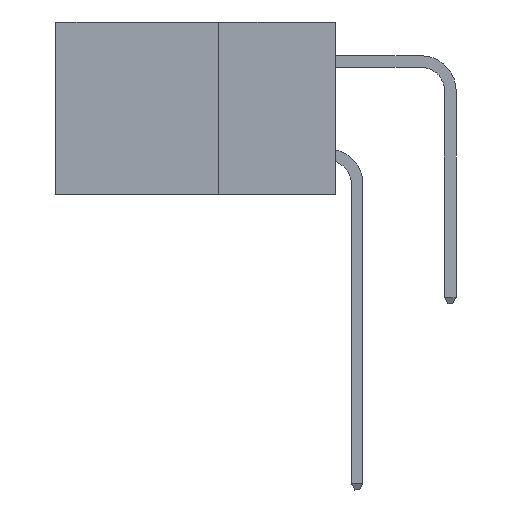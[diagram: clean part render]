
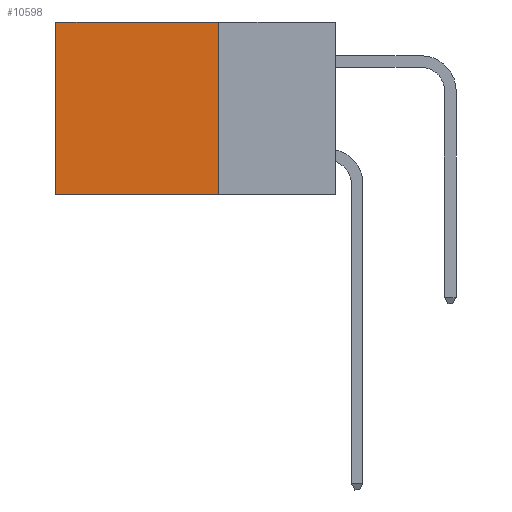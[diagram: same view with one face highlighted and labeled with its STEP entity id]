
A CAD part, left-side view. The second image highlights one B-rep face of the part: STEP entity #10598.
In plain terms, the highlighted planar face has unit normal (-1, 0, 0).
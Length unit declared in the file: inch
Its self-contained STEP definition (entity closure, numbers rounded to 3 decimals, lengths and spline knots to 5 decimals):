
#265 = ORIENTED_EDGE ( 'NONE', *, *, #7087, .T. ) ;
#295 = CARTESIAN_POINT ( 'NONE',  ( 0.2875, 0.6, 0. ) ) ;
#411 = VERTEX_POINT ( 'NONE', #9267 ) ;
#1219 = DIRECTION ( 'NONE',  ( 1., 0., 0. ) ) ;
#1471 = ORIENTED_EDGE ( 'NONE', *, *, #13299, .F. ) ;
#1819 = DIRECTION ( 'NONE',  ( 0., 0., -1. ) ) ;
#2001 = CARTESIAN_POINT ( 'NONE',  ( 0.2875, 0.6, 0. ) ) ;
#3094 = VECTOR ( 'NONE', #5491, 39.37008 ) ;
#3588 = CARTESIAN_POINT ( 'NONE',  ( 0.2875, 0.25, -0.37 ) ) ;
#3976 = CARTESIAN_POINT ( 'NONE',  ( 0.2875, 0.25, -0.37 ) ) ;
#4157 = CARTESIAN_POINT ( 'NONE',  ( 0.2875, 0.25, 0. ) ) ;
#5035 = VERTEX_POINT ( 'NONE', #4157 ) ;
#5067 = LINE ( 'NONE', #17633, #13308 ) ;
#5439 = VERTEX_POINT ( 'NONE', #2001 ) ;
#5491 = DIRECTION ( 'NONE',  ( 0., 1., 0. ) ) ;
#6133 = DIRECTION ( 'NONE',  ( 0., 0., -1. ) ) ;
#6838 = DIRECTION ( 'NONE',  ( 0., 1., 0. ) ) ;
#7087 = EDGE_CURVE ( 'NONE', #5035, #5439, #5067, .T. ) ;
#7110 = VECTOR ( 'NONE', #6133, 39.37008 ) ;
#8723 = VECTOR ( 'NONE', #1819, 39.37008 ) ;
#8819 = PLANE ( 'NONE',  #9483 ) ;
#9163 = EDGE_CURVE ( 'NONE', #5035, #13132, #11830, .T. ) ;
#9267 = CARTESIAN_POINT ( 'NONE',  ( 0.2875, 0.6, -0.37 ) ) ;
#9483 = AXIS2_PLACEMENT_3D ( 'NONE', #19409, #1219, #12051 ) ;
#9643 = ORIENTED_EDGE ( 'NONE', *, *, #9163, .F. ) ;
#10598 = ADVANCED_FACE ( 'NONE', ( #18038 ), #8819, .F. ) ;
#11371 = LINE ( 'NONE', #3976, #3094 ) ;
#11830 = LINE ( 'NONE', #15481, #7110 ) ;
#12051 = DIRECTION ( 'NONE',  ( 0., 0., -1. ) ) ;
#13132 = VERTEX_POINT ( 'NONE', #3588 ) ;
#13299 = EDGE_CURVE ( 'NONE', #13132, #411, #11371, .T. ) ;
#13308 = VECTOR ( 'NONE', #6838, 39.37008 ) ;
#13607 = ORIENTED_EDGE ( 'NONE', *, *, #15523, .T. ) ;
#15481 = CARTESIAN_POINT ( 'NONE',  ( 0.2875, 0.25, 0. ) ) ;
#15523 = EDGE_CURVE ( 'NONE', #5439, #411, #17330, .T. ) ;
#16524 = EDGE_LOOP ( 'NONE', ( #13607, #1471, #9643, #265 ) ) ;
#17330 = LINE ( 'NONE', #295, #8723 ) ;
#17633 = CARTESIAN_POINT ( 'NONE',  ( 0.2875, 0.25, 0. ) ) ;
#18038 = FACE_OUTER_BOUND ( 'NONE', #16524, .T. ) ;
#19409 = CARTESIAN_POINT ( 'NONE',  ( 0.2875, 0.25, 0. ) ) ;
